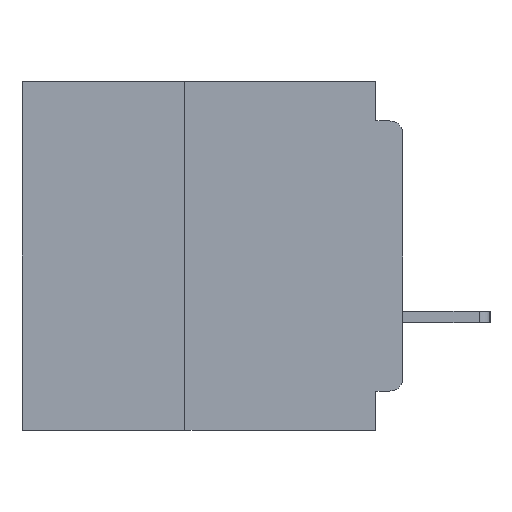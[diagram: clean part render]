
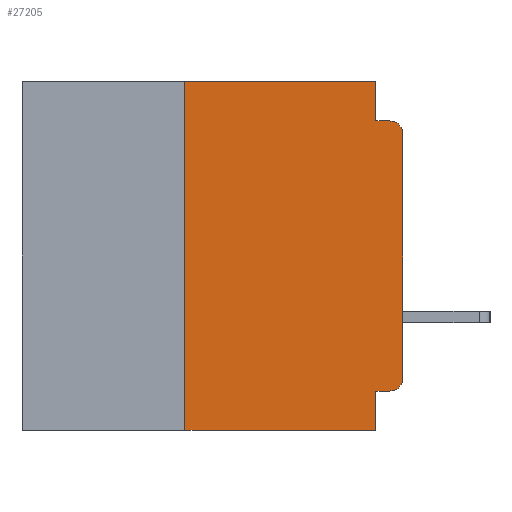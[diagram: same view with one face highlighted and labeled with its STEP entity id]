
A CAD part, left-side view. The second image highlights one B-rep face of the part: STEP entity #27205.
In plain terms, the highlighted planar face has unit normal (-1, 0, 0).
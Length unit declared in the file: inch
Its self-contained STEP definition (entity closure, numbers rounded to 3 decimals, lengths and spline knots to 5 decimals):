
#2231 = DIRECTION ( 'NONE',  ( 0., 0., 1. ) ) ;
#4314 = VERTEX_POINT ( 'NONE', #19278 ) ;
#5197 = EDGE_CURVE ( 'NONE', #8638, #47262, #45402, .T. ) ;
#6221 = ORIENTED_EDGE ( 'NONE', *, *, #47217, .F. ) ;
#6891 = DIRECTION ( 'NONE',  ( 0., -1., 0. ) ) ;
#7090 = ORIENTED_EDGE ( 'NONE', *, *, #5197, .T. ) ;
#7526 = CARTESIAN_POINT ( 'NONE',  ( 0., 0.031, -0.4 ) ) ;
#7853 = LINE ( 'NONE', #44962, #42671 ) ;
#8411 = LINE ( 'NONE', #16468, #33660 ) ;
#8638 = VERTEX_POINT ( 'NONE', #19134 ) ;
#8743 = DIRECTION ( 'NONE',  ( 0., -1., 0. ) ) ;
#8860 = CIRCLE ( 'NONE', #24418, 0.015 ) ;
#10958 = CARTESIAN_POINT ( 'NONE',  ( 0., 0.031, -0.355 ) ) ;
#11255 = LINE ( 'NONE', #49483, #59978 ) ;
#12167 = VERTEX_POINT ( 'NONE', #7526 ) ;
#12210 = CARTESIAN_POINT ( 'NONE',  ( 0., 0.25, -0.4 ) ) ;
#12313 = EDGE_CURVE ( 'NONE', #50832, #12167, #56595, .T. ) ;
#12816 = CARTESIAN_POINT ( 'NONE',  ( 0., 0.25, 0. ) ) ;
#13137 = VERTEX_POINT ( 'NONE', #10958 ) ;
#13489 = DIRECTION ( 'NONE',  ( -1., 0., 0. ) ) ;
#13531 = CARTESIAN_POINT ( 'NONE',  ( 0., 0.437, -0.4 ) ) ;
#16243 = EDGE_CURVE ( 'NONE', #47262, #59239, #8860, .T. ) ;
#16303 = EDGE_CURVE ( 'NONE', #17985, #59149, #54702, .T. ) ;
#16468 = CARTESIAN_POINT ( 'NONE',  ( 0., 0., -0.045 ) ) ;
#16616 = CARTESIAN_POINT ( 'NONE',  ( 0., 0., -0.06 ) ) ;
#17159 = EDGE_CURVE ( 'NONE', #4314, #13137, #18392, .T. ) ;
#17985 = VERTEX_POINT ( 'NONE', #20764 ) ;
#18392 = LINE ( 'NONE', #44516, #42064 ) ;
#18527 = VECTOR ( 'NONE', #47706, 39.37008 ) ;
#18893 = ORIENTED_EDGE ( 'NONE', *, *, #27259, .F. ) ;
#19134 = CARTESIAN_POINT ( 'NONE',  ( 0., 0., -0.34 ) ) ;
#19278 = CARTESIAN_POINT ( 'NONE',  ( 0., 0.015, -0.355 ) ) ;
#20650 = CARTESIAN_POINT ( 'NONE',  ( 0., 0.437, 0. ) ) ;
#20764 = CARTESIAN_POINT ( 'NONE',  ( 0., 0.031, 0. ) ) ;
#21201 = DIRECTION ( 'NONE',  ( 0., -1., 0. ) ) ;
#21770 = VECTOR ( 'NONE', #44985, 39.37008 ) ;
#24418 = AXIS2_PLACEMENT_3D ( 'NONE', #56724, #28529, #61410 ) ;
#25387 = DIRECTION ( 'NONE',  ( 0., 0., -1. ) ) ;
#27155 = CARTESIAN_POINT ( 'NONE',  ( 0., 0.031, -0.4 ) ) ;
#27205 = ADVANCED_FACE ( 'NONE', ( #49163 ), #34696, .F. ) ;
#27259 = EDGE_CURVE ( 'NONE', #59149, #59239, #8411, .T. ) ;
#27265 = ORIENTED_EDGE ( 'NONE', *, *, #12313, .T. ) ;
#28529 = DIRECTION ( 'NONE',  ( -1., 0., 0. ) ) ;
#29076 = ORIENTED_EDGE ( 'NONE', *, *, #16303, .F. ) ;
#29730 = CIRCLE ( 'NONE', #34294, 0.015 ) ;
#31279 = ORIENTED_EDGE ( 'NONE', *, *, #48566, .T. ) ;
#31917 = DIRECTION ( 'NONE',  ( 0., 0., -1. ) ) ;
#33660 = VECTOR ( 'NONE', #6891, 39.37008 ) ;
#34294 = AXIS2_PLACEMENT_3D ( 'NONE', #41837, #13489, #46583 ) ;
#34696 = PLANE ( 'NONE',  #50972 ) ;
#39785 = DIRECTION ( 'NONE',  ( 0., 1., 0. ) ) ;
#40254 = CARTESIAN_POINT ( 'NONE',  ( 0., 0., 0. ) ) ;
#40452 = CARTESIAN_POINT ( 'NONE',  ( 0., 0.031, -0.045 ) ) ;
#41837 = CARTESIAN_POINT ( 'NONE',  ( 0., 0.015, -0.34 ) ) ;
#42064 = VECTOR ( 'NONE', #39785, 39.37008 ) ;
#42671 = VECTOR ( 'NONE', #2231, 39.37008 ) ;
#42962 = CARTESIAN_POINT ( 'NONE',  ( 0., 0.031, 0. ) ) ;
#43340 = ORIENTED_EDGE ( 'NONE', *, *, #54101, .F. ) ;
#44109 = VECTOR ( 'NONE', #8743, 39.37008 ) ;
#44516 = CARTESIAN_POINT ( 'NONE',  ( 0., 0., -0.355 ) ) ;
#44962 = CARTESIAN_POINT ( 'NONE',  ( 0., 0.25, -0.4 ) ) ;
#44985 = DIRECTION ( 'NONE',  ( 0., 0., 1. ) ) ;
#45171 = VECTOR ( 'NONE', #31917, 39.37008 ) ;
#45402 = LINE ( 'NONE', #40254, #21770 ) ;
#46583 = DIRECTION ( 'NONE',  ( 0., 0., -1. ) ) ;
#47217 = EDGE_CURVE ( 'NONE', #47893, #17985, #11255, .T. ) ;
#47262 = VERTEX_POINT ( 'NONE', #16616 ) ;
#47706 = DIRECTION ( 'NONE',  ( 0., 0., -1. ) ) ;
#47893 = VERTEX_POINT ( 'NONE', #12816 ) ;
#48566 = EDGE_CURVE ( 'NONE', #4314, #8638, #29730, .T. ) ;
#49163 = FACE_OUTER_BOUND ( 'NONE', #51211, .T. ) ;
#49383 = ORIENTED_EDGE ( 'NONE', *, *, #17159, .F. ) ;
#49483 = CARTESIAN_POINT ( 'NONE',  ( 0., 0.437, 0. ) ) ;
#50183 = EDGE_CURVE ( 'NONE', #50832, #47893, #7853, .T. ) ;
#50343 = ORIENTED_EDGE ( 'NONE', *, *, #50183, .F. ) ;
#50832 = VERTEX_POINT ( 'NONE', #12210 ) ;
#50972 = AXIS2_PLACEMENT_3D ( 'NONE', #20650, #53621, #25387 ) ;
#51211 = EDGE_LOOP ( 'NONE', ( #7090, #59560, #18893, #29076, #6221, #50343, #27265, #43340, #49383, #31279 ) ) ;
#53621 = DIRECTION ( 'NONE',  ( 1., 0., 0. ) ) ;
#54101 = EDGE_CURVE ( 'NONE', #13137, #12167, #59118, .T. ) ;
#54702 = LINE ( 'NONE', #42962, #18527 ) ;
#56595 = LINE ( 'NONE', #13531, #44109 ) ;
#56724 = CARTESIAN_POINT ( 'NONE',  ( 0., 0.015, -0.06 ) ) ;
#59118 = LINE ( 'NONE', #27155, #45171 ) ;
#59149 = VERTEX_POINT ( 'NONE', #40452 ) ;
#59239 = VERTEX_POINT ( 'NONE', #59927 ) ;
#59560 = ORIENTED_EDGE ( 'NONE', *, *, #16243, .T. ) ;
#59927 = CARTESIAN_POINT ( 'NONE',  ( 0., 0.015, -0.045 ) ) ;
#59978 = VECTOR ( 'NONE', #21201, 39.37008 ) ;
#61410 = DIRECTION ( 'NONE',  ( 0., 0., -1. ) ) ;
